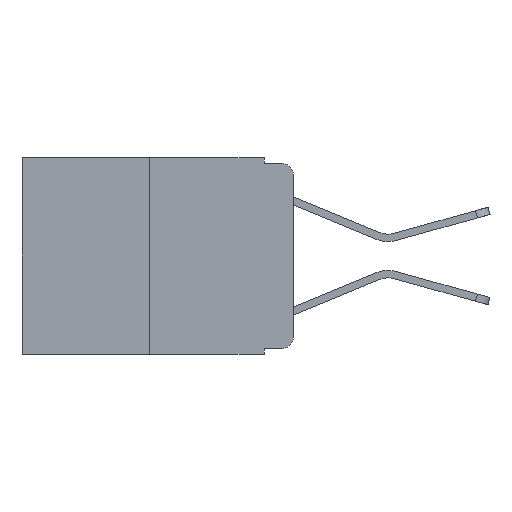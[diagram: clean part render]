
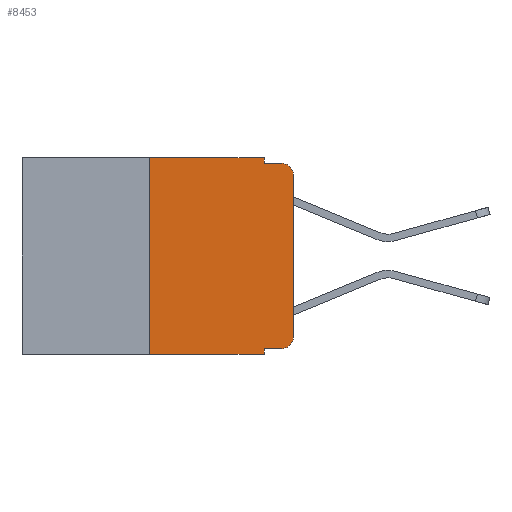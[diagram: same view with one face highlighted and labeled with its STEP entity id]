
A CAD part, left-side view. The second image highlights one B-rep face of the part: STEP entity #8453.
In plain terms, the highlighted planar face has unit normal (-1, 0, 0).
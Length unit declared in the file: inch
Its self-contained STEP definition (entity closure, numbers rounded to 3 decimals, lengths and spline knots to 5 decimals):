
#196 = VERTEX_POINT ( 'NONE', #4408 ) ;
#296 = DIRECTION ( 'NONE',  ( 0., -1., 0. ) ) ;
#434 = VERTEX_POINT ( 'NONE', #6528 ) ;
#465 = LINE ( 'NONE', #13832, #9843 ) ;
#582 = ORIENTED_EDGE ( 'NONE', *, *, #8480, .T. ) ;
#630 = ORIENTED_EDGE ( 'NONE', *, *, #5497, .F. ) ;
#715 = ORIENTED_EDGE ( 'NONE', *, *, #7736, .T. ) ;
#797 = CARTESIAN_POINT ( 'NONE',  ( 0., 0.051, 0. ) ) ;
#820 = DIRECTION ( 'NONE',  ( 0., -1., 0. ) ) ;
#881 = ORIENTED_EDGE ( 'NONE', *, *, #6996, .F. ) ;
#946 = DIRECTION ( 'NONE',  ( 0., 0., 1. ) ) ;
#1096 = DIRECTION ( 'NONE',  ( 0., 0., -1. ) ) ;
#1117 = ORIENTED_EDGE ( 'NONE', *, *, #6262, .F. ) ;
#1311 = ORIENTED_EDGE ( 'NONE', *, *, #5419, .F. ) ;
#1341 = DIRECTION ( 'NONE',  ( 1., 0., 0. ) ) ;
#1424 = CARTESIAN_POINT ( 'NONE',  ( 0., 0.051, -0.343 ) ) ;
#1575 = ORIENTED_EDGE ( 'NONE', *, *, #9707, .T. ) ;
#1878 = LINE ( 'NONE', #14806, #10929 ) ;
#2316 = CARTESIAN_POINT ( 'NONE',  ( 0., 0.25, 0. ) ) ;
#2933 = LINE ( 'NONE', #7570, #14610 ) ;
#3004 = EDGE_CURVE ( 'NONE', #8537, #196, #13655, .T. ) ;
#3050 = VERTEX_POINT ( 'NONE', #14190 ) ;
#3053 = VERTEX_POINT ( 'NONE', #1424 ) ;
#3865 = EDGE_CURVE ( 'NONE', #3050, #8537, #465, .T. ) ;
#3876 = CARTESIAN_POINT ( 'NONE',  ( 0., 0.051, 0. ) ) ;
#3953 = VECTOR ( 'NONE', #296, 39.37008 ) ;
#4120 = DIRECTION ( 'NONE',  ( 0., 0., 1. ) ) ;
#4307 = DIRECTION ( 'NONE',  ( -1., 0., 0. ) ) ;
#4375 = CARTESIAN_POINT ( 'NONE',  ( 0., 0.02, -0.01 ) ) ;
#4408 = CARTESIAN_POINT ( 'NONE',  ( 0., 0., -0.313 ) ) ;
#4741 = EDGE_CURVE ( 'NONE', #3050, #3053, #8153, .T. ) ;
#4827 = VERTEX_POINT ( 'NONE', #6366 ) ;
#5022 = DIRECTION ( 'NONE',  ( 0., -1., 0. ) ) ;
#5400 = EDGE_LOOP ( 'NONE', ( #582, #715, #881, #1117, #1311, #630, #1575, #5463, #13228, #11480 ) ) ;
#5419 = EDGE_CURVE ( 'NONE', #11713, #434, #1878, .T. ) ;
#5434 = CARTESIAN_POINT ( 'NONE',  ( 0., 0.02, -0.333 ) ) ;
#5463 = ORIENTED_EDGE ( 'NONE', *, *, #4741, .F. ) ;
#5497 = EDGE_CURVE ( 'NONE', #11794, #11713, #13157, .T. ) ;
#5518 = AXIS2_PLACEMENT_3D ( 'NONE', #10854, #1341, #9769 ) ;
#5860 = LINE ( 'NONE', #797, #8449 ) ;
#6155 = CARTESIAN_POINT ( 'NONE',  ( 0., 0.473, -0.343 ) ) ;
#6186 = FACE_OUTER_BOUND ( 'NONE', #5400, .T. ) ;
#6262 = EDGE_CURVE ( 'NONE', #434, #4827, #5860, .T. ) ;
#6366 = CARTESIAN_POINT ( 'NONE',  ( 0., 0.051, -0.01 ) ) ;
#6468 = VERTEX_POINT ( 'NONE', #8451 ) ;
#6528 = CARTESIAN_POINT ( 'NONE',  ( 0., 0.051, 0. ) ) ;
#6996 = EDGE_CURVE ( 'NONE', #4827, #12869, #7385, .T. ) ;
#7385 = LINE ( 'NONE', #10098, #3953 ) ;
#7489 = DIRECTION ( 'NONE',  ( -1., 0., 0. ) ) ;
#7570 = CARTESIAN_POINT ( 'NONE',  ( 0., 0., 0. ) ) ;
#7736 = EDGE_CURVE ( 'NONE', #6468, #12869, #10199, .T. ) ;
#7798 = VECTOR ( 'NONE', #1096, 39.37008 ) ;
#8153 = LINE ( 'NONE', #3876, #7798 ) ;
#8227 = LINE ( 'NONE', #6155, #13754 ) ;
#8337 = CARTESIAN_POINT ( 'NONE',  ( 0., 0.25, 0. ) ) ;
#8353 = AXIS2_PLACEMENT_3D ( 'NONE', #14103, #7489, #15150 ) ;
#8449 = VECTOR ( 'NONE', #10473, 39.37008 ) ;
#8451 = CARTESIAN_POINT ( 'NONE',  ( 0., 0., -0.03 ) ) ;
#8453 = ADVANCED_FACE ( 'NONE', ( #6186 ), #8637, .F. ) ;
#8480 = EDGE_CURVE ( 'NONE', #196, #6468, #2933, .T. ) ;
#8537 = VERTEX_POINT ( 'NONE', #5434 ) ;
#8637 = PLANE ( 'NONE',  #5518 ) ;
#9681 = CARTESIAN_POINT ( 'NONE',  ( 0., 0.25, -0.343 ) ) ;
#9707 = EDGE_CURVE ( 'NONE', #11794, #3053, #8227, .T. ) ;
#9769 = DIRECTION ( 'NONE',  ( 0., 0., -1. ) ) ;
#9843 = VECTOR ( 'NONE', #5022, 39.37008 ) ;
#10096 = AXIS2_PLACEMENT_3D ( 'NONE', #11046, #4307, #12153 ) ;
#10098 = CARTESIAN_POINT ( 'NONE',  ( 0., 0.051, -0.01 ) ) ;
#10199 = CIRCLE ( 'NONE', #10096, 0.02 ) ;
#10473 = DIRECTION ( 'NONE',  ( 0., 0., -1. ) ) ;
#10585 = VECTOR ( 'NONE', #946, 39.37008 ) ;
#10854 = CARTESIAN_POINT ( 'NONE',  ( 0., 0.473, 0. ) ) ;
#10929 = VECTOR ( 'NONE', #820, 39.37008 ) ;
#11046 = CARTESIAN_POINT ( 'NONE',  ( 0., 0.02, -0.03 ) ) ;
#11480 = ORIENTED_EDGE ( 'NONE', *, *, #3004, .T. ) ;
#11669 = DIRECTION ( 'NONE',  ( 0., -1., 0. ) ) ;
#11713 = VERTEX_POINT ( 'NONE', #2316 ) ;
#11794 = VERTEX_POINT ( 'NONE', #9681 ) ;
#12153 = DIRECTION ( 'NONE',  ( 0., 0., -1. ) ) ;
#12869 = VERTEX_POINT ( 'NONE', #4375 ) ;
#13157 = LINE ( 'NONE', #8337, #10585 ) ;
#13228 = ORIENTED_EDGE ( 'NONE', *, *, #3865, .T. ) ;
#13655 = CIRCLE ( 'NONE', #8353, 0.02 ) ;
#13754 = VECTOR ( 'NONE', #11669, 39.37008 ) ;
#13832 = CARTESIAN_POINT ( 'NONE',  ( 0., 0.051, -0.333 ) ) ;
#14103 = CARTESIAN_POINT ( 'NONE',  ( 0., 0.02, -0.313 ) ) ;
#14190 = CARTESIAN_POINT ( 'NONE',  ( 0., 0.051, -0.333 ) ) ;
#14610 = VECTOR ( 'NONE', #4120, 39.37008 ) ;
#14806 = CARTESIAN_POINT ( 'NONE',  ( 0., 0.473, 0. ) ) ;
#15150 = DIRECTION ( 'NONE',  ( 0., 0., -1. ) ) ;
